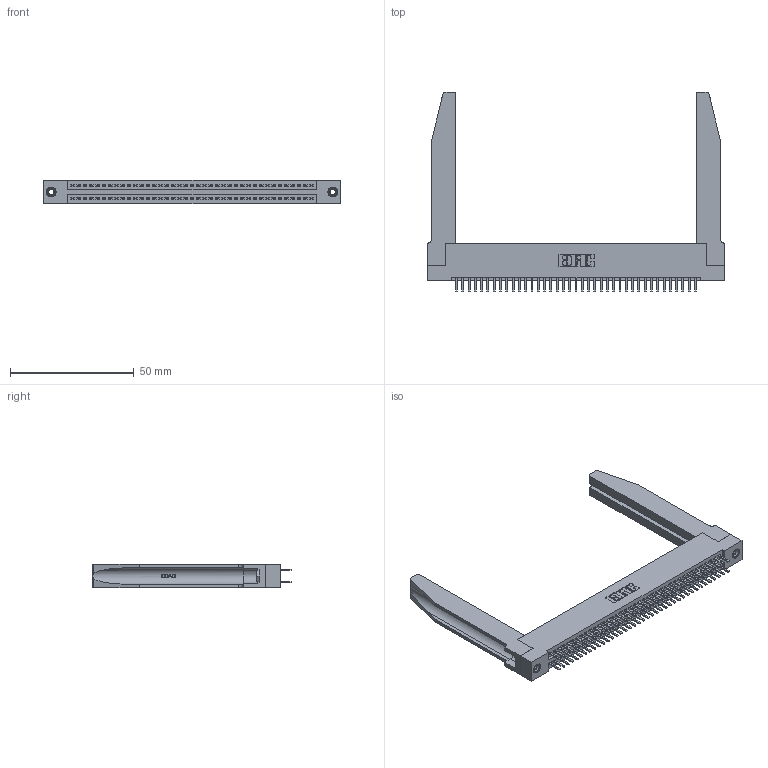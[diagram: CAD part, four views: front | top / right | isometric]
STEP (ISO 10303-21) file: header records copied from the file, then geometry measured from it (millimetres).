
FILE_DESCRIPTION (( 'STEP AP203' ), '1' );
FILE_NAME ('395-078-520-278.STEP', '2019-10-24T18:09:22', ( '' ), ( '' ), 'SwSTEP 2.0', 'SolidWorks 2016', '' );
FILE_SCHEMA (( 'CONFIG_CONTROL_DESIGN' ));
Length unit declared in the file: inch
Products named in the file (5): 345 Part_Flush Mounting Lugs - 0.156 Dia-TH; 345-292-001_345-293-120; 345-250-001_345-250-001-102; 345-220-078_345-220-078; 395-078-520-278
Assembly tree (83 placements, depth 2):
  395-078-520-278
    345 Part_Flush Mounting Lugs - 0.156 Dia-TH
    345-292-001_345-293-120  x78
    345-250-001_345-250-001-102  x2
    345-220-078_345-220-078  x2
Bounding box: 120.29 x 80.64 x 9.4 mm (x, y, z)
Volume: 19393.8 mm3; surface area: 23888.7 mm2
Topology: 83 solids, 83 shells, 4572 faces, 13195 edges, 8578 vertices
Faces by surface type: plane 2952, cylinder 1568, bspline 36, cone 12, torus 4
Entity records: 35858 total; most frequent: CARTESIAN_POINT 6943, ORIENTED_EDGE 5762, DIRECTION 5107, EDGE_CURVE 2881, LINE 2495, VECTOR 2495, VERTEX_POINT 1912, AXIS2_PLACEMENT_3D 1306
